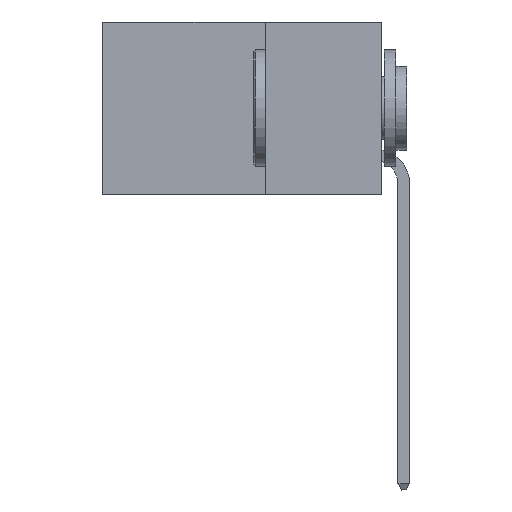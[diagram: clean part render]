
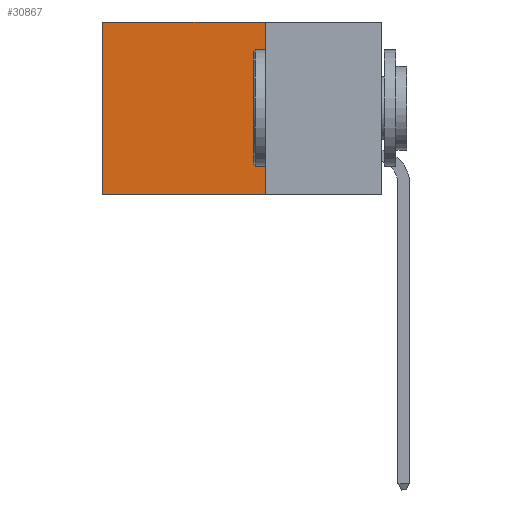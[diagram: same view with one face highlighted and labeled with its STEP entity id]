
A CAD part, left-side view. The second image highlights one B-rep face of the part: STEP entity #30867.
In plain terms, the highlighted planar face has unit normal (-1, 0, 0).
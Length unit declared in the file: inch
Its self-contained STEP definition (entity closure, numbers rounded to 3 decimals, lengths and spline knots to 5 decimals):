
#4231 = DIRECTION ( 'NONE',  ( 0., 1., 0. ) ) ;
#4777 = CARTESIAN_POINT ( 'NONE',  ( 0.2875, 0.25, -0.37 ) ) ;
#7163 = CARTESIAN_POINT ( 'NONE',  ( 0.2875, 0.25, 0. ) ) ;
#7342 = DIRECTION ( 'NONE',  ( 0., 0., -1. ) ) ;
#7912 = LINE ( 'NONE', #38095, #24941 ) ;
#11031 = ORIENTED_EDGE ( 'NONE', *, *, #37492, .F. ) ;
#11306 = EDGE_CURVE ( 'NONE', #36514, #31622, #32922, .T. ) ;
#12819 = EDGE_LOOP ( 'NONE', ( #37880, #15332, #11031, #36945 ) ) ;
#13493 = VERTEX_POINT ( 'NONE', #18626 ) ;
#15332 = ORIENTED_EDGE ( 'NONE', *, *, #11306, .F. ) ;
#17521 = LINE ( 'NONE', #40470, #34007 ) ;
#17617 = CARTESIAN_POINT ( 'NONE',  ( 0.2875, 0.25, 0. ) ) ;
#17793 = DIRECTION ( 'NONE',  ( 0., 0., -1. ) ) ;
#18626 = CARTESIAN_POINT ( 'NONE',  ( 0.2875, 0.6, 0. ) ) ;
#19165 = VECTOR ( 'NONE', #43441, 39.37008 ) ;
#19495 = VECTOR ( 'NONE', #4231, 39.37008 ) ;
#23651 = FACE_OUTER_BOUND ( 'NONE', #12819, .T. ) ;
#24585 = CARTESIAN_POINT ( 'NONE',  ( 0.2875, 0.25, 0. ) ) ;
#24941 = VECTOR ( 'NONE', #17793, 39.37008 ) ;
#27057 = DIRECTION ( 'NONE',  ( 0., 0., -1. ) ) ;
#27854 = AXIS2_PLACEMENT_3D ( 'NONE', #17617, #41557, #7342 ) ;
#27932 = VERTEX_POINT ( 'NONE', #7163 ) ;
#29769 = CARTESIAN_POINT ( 'NONE',  ( 0.2875, 0.25, -0.37 ) ) ;
#30867 = ADVANCED_FACE ( 'NONE', ( #23651 ), #37930, .F. ) ;
#31622 = VERTEX_POINT ( 'NONE', #38671 ) ;
#32922 = LINE ( 'NONE', #29769, #19165 ) ;
#34007 = VECTOR ( 'NONE', #27057, 39.37008 ) ;
#36514 = VERTEX_POINT ( 'NONE', #4777 ) ;
#36725 = EDGE_CURVE ( 'NONE', #13493, #31622, #17521, .T. ) ;
#36945 = ORIENTED_EDGE ( 'NONE', *, *, #39689, .T. ) ;
#37484 = LINE ( 'NONE', #24585, #19495 ) ;
#37492 = EDGE_CURVE ( 'NONE', #27932, #36514, #7912, .T. ) ;
#37880 = ORIENTED_EDGE ( 'NONE', *, *, #36725, .T. ) ;
#37930 = PLANE ( 'NONE',  #27854 ) ;
#38095 = CARTESIAN_POINT ( 'NONE',  ( 0.2875, 0.25, 0. ) ) ;
#38671 = CARTESIAN_POINT ( 'NONE',  ( 0.2875, 0.6, -0.37 ) ) ;
#39689 = EDGE_CURVE ( 'NONE', #27932, #13493, #37484, .T. ) ;
#40470 = CARTESIAN_POINT ( 'NONE',  ( 0.2875, 0.6, 0. ) ) ;
#41557 = DIRECTION ( 'NONE',  ( 1., 0., 0. ) ) ;
#43441 = DIRECTION ( 'NONE',  ( 0., 1., 0. ) ) ;
